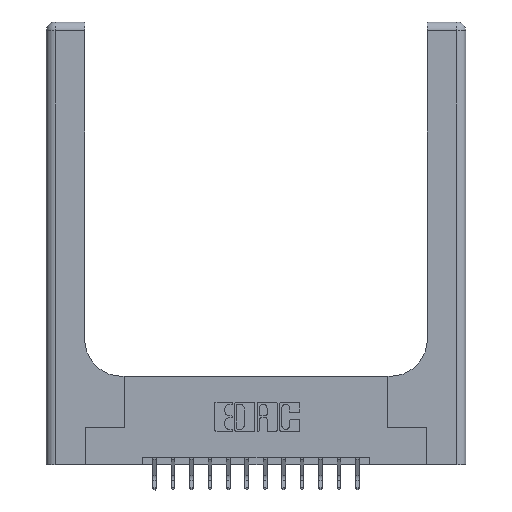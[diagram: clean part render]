
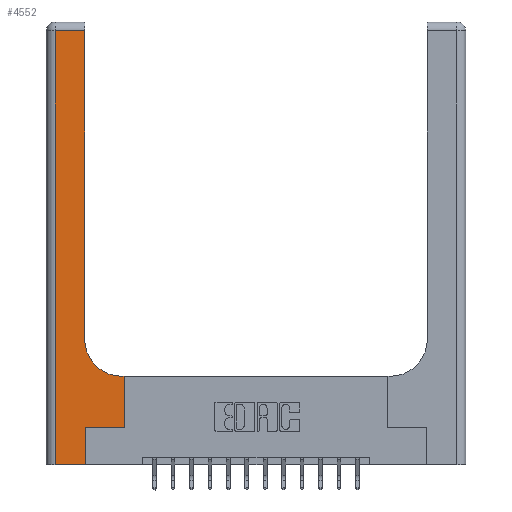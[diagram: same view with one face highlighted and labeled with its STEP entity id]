
A CAD part, top view. The second image highlights one B-rep face of the part: STEP entity #4552.
In plain terms, the highlighted planar face has unit normal (0, 0, 1).
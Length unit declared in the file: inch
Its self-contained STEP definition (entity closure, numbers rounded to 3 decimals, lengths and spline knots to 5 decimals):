
#156 = ORIENTED_EDGE ( 'NONE', *, *, #12272, .T. ) ;
#161 = EDGE_LOOP ( 'NONE', ( #12472, #6544, #10709, #806, #10929, #4544, #156, #7984, #10786 ) ) ;
#550 = CARTESIAN_POINT ( 'NONE',  ( 0.265, 0.25, 0.37 ) ) ;
#605 = CARTESIAN_POINT ( 'NONE',  ( 0.265, 0., 0.37 ) ) ;
#615 = VECTOR ( 'NONE', #2563, 39.37008 ) ;
#806 = ORIENTED_EDGE ( 'NONE', *, *, #16758, .T. ) ;
#991 = DIRECTION ( 'NONE',  ( 0., 1., 0. ) ) ;
#1356 = VECTOR ( 'NONE', #991, 39.37008 ) ;
#1462 = LINE ( 'NONE', #2192, #615 ) ;
#1484 = LINE ( 'NONE', #7281, #8573 ) ;
#1603 = EDGE_CURVE ( 'NONE', #8721, #13671, #12405, .T. ) ;
#1758 = LINE ( 'NONE', #10318, #14940 ) ;
#1851 = VERTEX_POINT ( 'NONE', #12563 ) ;
#2192 = CARTESIAN_POINT ( 'NONE',  ( 0.26, 0.6, 0.37 ) ) ;
#2494 = CARTESIAN_POINT ( 'NONE',  ( 0.26, 0.85, 0.37 ) ) ;
#2563 = DIRECTION ( 'NONE',  ( -1., 0., 0. ) ) ;
#2641 = CARTESIAN_POINT ( 'NONE',  ( 0.528, 0.6, 0.37 ) ) ;
#2685 = VECTOR ( 'NONE', #7728, 39.37008 ) ;
#2765 = LINE ( 'NONE', #15010, #9407 ) ;
#2937 = LINE ( 'NONE', #7875, #4423 ) ;
#3139 = DIRECTION ( 'NONE',  ( 0., 1., 0. ) ) ;
#3944 = DIRECTION ( 'NONE',  ( 1., 0., 0. ) ) ;
#3956 = EDGE_CURVE ( 'NONE', #13328, #8721, #1462, .T. ) ;
#4051 = VERTEX_POINT ( 'NONE', #7760 ) ;
#4423 = VECTOR ( 'NONE', #3944, 39.37008 ) ;
#4544 = ORIENTED_EDGE ( 'NONE', *, *, #17115, .T. ) ;
#4552 = ADVANCED_FACE ( 'NONE', ( #8133 ), #13271, .F. ) ;
#4612 = AXIS2_PLACEMENT_3D ( 'NONE', #9078, #7882, #6621 ) ;
#5771 = DIRECTION ( 'NONE',  ( 1., 0., 0. ) ) ;
#6121 = CARTESIAN_POINT ( 'NONE',  ( 0.06, 2.94, 0.37 ) ) ;
#6542 = EDGE_CURVE ( 'NONE', #8825, #7053, #1758, .T. ) ;
#6544 = ORIENTED_EDGE ( 'NONE', *, *, #8184, .T. ) ;
#6621 = DIRECTION ( 'NONE',  ( -1., 0., 0. ) ) ;
#7044 = DIRECTION ( 'NONE',  ( 0., -1., 0. ) ) ;
#7053 = VERTEX_POINT ( 'NONE', #13046 ) ;
#7169 = CARTESIAN_POINT ( 'NONE',  ( 0.51, 0.85, 0.37 ) ) ;
#7243 = EDGE_CURVE ( 'NONE', #13671, #10380, #14102, .T. ) ;
#7281 = CARTESIAN_POINT ( 'NONE',  ( 0.528, 0.25, 0.37 ) ) ;
#7479 = DIRECTION ( 'NONE',  ( 0., 1., 0. ) ) ;
#7663 = CARTESIAN_POINT ( 'NONE',  ( 0., 2.94, 0.37 ) ) ;
#7680 = CARTESIAN_POINT ( 'NONE',  ( 0.26, 2.94, 0.37 ) ) ;
#7728 = DIRECTION ( 'NONE',  ( -1., 0., 0. ) ) ;
#7760 = CARTESIAN_POINT ( 'NONE',  ( 0.528, 0.25, 0.37 ) ) ;
#7875 = CARTESIAN_POINT ( 'NONE',  ( 0., 0., 0.37 ) ) ;
#7882 = DIRECTION ( 'NONE',  ( 0., 0., -1. ) ) ;
#7971 = AXIS2_PLACEMENT_3D ( 'NONE', #7169, #11115, #14016 ) ;
#7984 = ORIENTED_EDGE ( 'NONE', *, *, #3956, .T. ) ;
#8133 = FACE_OUTER_BOUND ( 'NONE', #161, .T. ) ;
#8184 = EDGE_CURVE ( 'NONE', #10380, #8921, #16439, .T. ) ;
#8573 = VECTOR ( 'NONE', #3139, 39.37008 ) ;
#8721 = VERTEX_POINT ( 'NONE', #16944 ) ;
#8825 = VERTEX_POINT ( 'NONE', #605 ) ;
#8921 = VERTEX_POINT ( 'NONE', #6121 ) ;
#9078 = CARTESIAN_POINT ( 'NONE',  ( 0., 3., 0.37 ) ) ;
#9363 = VECTOR ( 'NONE', #5771, 39.37008 ) ;
#9407 = VECTOR ( 'NONE', #7044, 39.37008 ) ;
#9792 = LINE ( 'NONE', #550, #9363 ) ;
#10318 = CARTESIAN_POINT ( 'NONE',  ( 0.265, 0., 0.37 ) ) ;
#10380 = VERTEX_POINT ( 'NONE', #7680 ) ;
#10709 = ORIENTED_EDGE ( 'NONE', *, *, #12453, .T. ) ;
#10786 = ORIENTED_EDGE ( 'NONE', *, *, #1603, .T. ) ;
#10929 = ORIENTED_EDGE ( 'NONE', *, *, #6542, .T. ) ;
#11115 = DIRECTION ( 'NONE',  ( 0., 0., -1. ) ) ;
#12272 = EDGE_CURVE ( 'NONE', #4051, #13328, #1484, .T. ) ;
#12405 = CIRCLE ( 'NONE', #7971, 0.25 ) ;
#12453 = EDGE_CURVE ( 'NONE', #8921, #1851, #2765, .T. ) ;
#12472 = ORIENTED_EDGE ( 'NONE', *, *, #7243, .T. ) ;
#12563 = CARTESIAN_POINT ( 'NONE',  ( 0.06, 0., 0.37 ) ) ;
#13046 = CARTESIAN_POINT ( 'NONE',  ( 0.265, 0.25, 0.37 ) ) ;
#13271 = PLANE ( 'NONE',  #4612 ) ;
#13328 = VERTEX_POINT ( 'NONE', #2641 ) ;
#13671 = VERTEX_POINT ( 'NONE', #2494 ) ;
#14016 = DIRECTION ( 'NONE',  ( 1., 0., 0. ) ) ;
#14102 = LINE ( 'NONE', #16995, #1356 ) ;
#14940 = VECTOR ( 'NONE', #7479, 39.37008 ) ;
#15010 = CARTESIAN_POINT ( 'NONE',  ( 0.06, 3., 0.37 ) ) ;
#16439 = LINE ( 'NONE', #7663, #2685 ) ;
#16758 = EDGE_CURVE ( 'NONE', #1851, #8825, #2937, .T. ) ;
#16944 = CARTESIAN_POINT ( 'NONE',  ( 0.51, 0.6, 0.37 ) ) ;
#16995 = CARTESIAN_POINT ( 'NONE',  ( 0.26, 3., 0.37 ) ) ;
#17115 = EDGE_CURVE ( 'NONE', #7053, #4051, #9792, .T. ) ;
